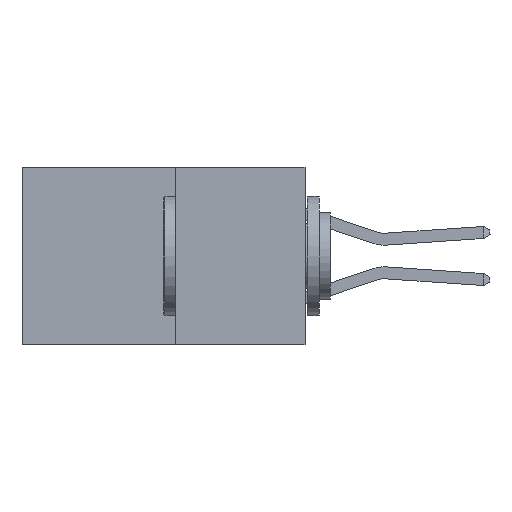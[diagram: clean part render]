
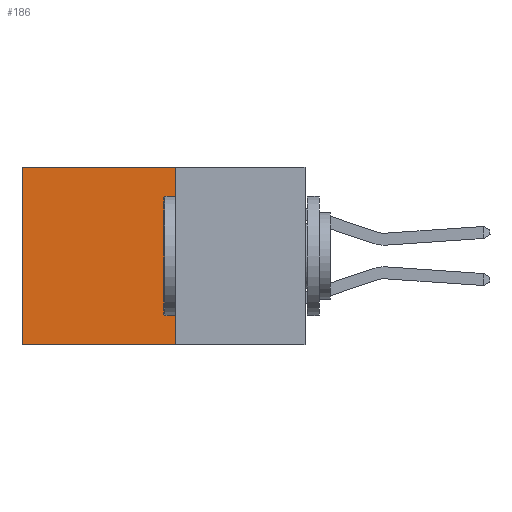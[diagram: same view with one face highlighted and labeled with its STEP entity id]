
A CAD part, left-side view. The second image highlights one B-rep face of the part: STEP entity #186.
In plain terms, the highlighted planar face has unit normal (-1, 0, 0).
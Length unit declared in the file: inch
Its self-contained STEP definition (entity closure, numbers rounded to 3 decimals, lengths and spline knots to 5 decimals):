
#186 = ADVANCED_FACE ( 'NONE', ( #20813 ), #20297, .F. ) ;
#725 = CARTESIAN_POINT ( 'NONE',  ( 0.277, 0.27, -0.37 ) ) ;
#1306 = ORIENTED_EDGE ( 'NONE', *, *, #22995, .F. ) ;
#1620 = CARTESIAN_POINT ( 'NONE',  ( 0.277, 0.27, 0. ) ) ;
#2730 = EDGE_CURVE ( 'NONE', #2996, #19503, #13261, .T. ) ;
#2996 = VERTEX_POINT ( 'NONE', #6154 ) ;
#4469 = ORIENTED_EDGE ( 'NONE', *, *, #5376, .T. ) ;
#4873 = CARTESIAN_POINT ( 'NONE',  ( 0.277, 0.27, -0.37 ) ) ;
#5376 = EDGE_CURVE ( 'NONE', #16649, #2996, #22531, .T. ) ;
#5715 = CARTESIAN_POINT ( 'NONE',  ( 0.277, 0.27, -0.37 ) ) ;
#6063 = LINE ( 'NONE', #5715, #15017 ) ;
#6154 = CARTESIAN_POINT ( 'NONE',  ( 0.277, 0.59, 0. ) ) ;
#6221 = DIRECTION ( 'NONE',  ( 0., 1., 0. ) ) ;
#6441 = ORIENTED_EDGE ( 'NONE', *, *, #13514, .F. ) ;
#6690 = LINE ( 'NONE', #725, #20286 ) ;
#6985 = CARTESIAN_POINT ( 'NONE',  ( 0.277, 0.27, 0. ) ) ;
#8928 = ORIENTED_EDGE ( 'NONE', *, *, #2730, .T. ) ;
#13236 = VECTOR ( 'NONE', #21013, 39.37008 ) ;
#13261 = LINE ( 'NONE', #19682, #17966 ) ;
#13514 = EDGE_CURVE ( 'NONE', #16649, #16453, #6063, .T. ) ;
#13796 = DIRECTION ( 'NONE',  ( 0., 0., -1. ) ) ;
#14583 = EDGE_LOOP ( 'NONE', ( #8928, #1306, #6441, #4469 ) ) ;
#15017 = VECTOR ( 'NONE', #16448, 39.37008 ) ;
#15549 = CARTESIAN_POINT ( 'NONE',  ( 0.277, 0.27, -0.37 ) ) ;
#16448 = DIRECTION ( 'NONE',  ( 0., 0., -1. ) ) ;
#16453 = VERTEX_POINT ( 'NONE', #15549 ) ;
#16649 = VERTEX_POINT ( 'NONE', #6985 ) ;
#16949 = AXIS2_PLACEMENT_3D ( 'NONE', #4873, #20514, #13796 ) ;
#17485 = DIRECTION ( 'NONE',  ( 0., 0., -1. ) ) ;
#17966 = VECTOR ( 'NONE', #17485, 39.37008 ) ;
#18236 = CARTESIAN_POINT ( 'NONE',  ( 0.277, 0.59, -0.37 ) ) ;
#19503 = VERTEX_POINT ( 'NONE', #18236 ) ;
#19682 = CARTESIAN_POINT ( 'NONE',  ( 0.277, 0.59, -0.37 ) ) ;
#20286 = VECTOR ( 'NONE', #6221, 39.37008 ) ;
#20297 = PLANE ( 'NONE',  #16949 ) ;
#20514 = DIRECTION ( 'NONE',  ( 1., 0., 0. ) ) ;
#20813 = FACE_OUTER_BOUND ( 'NONE', #14583, .T. ) ;
#21013 = DIRECTION ( 'NONE',  ( 0., 1., 0. ) ) ;
#22531 = LINE ( 'NONE', #1620, #13236 ) ;
#22995 = EDGE_CURVE ( 'NONE', #16453, #19503, #6690, .T. ) ;
